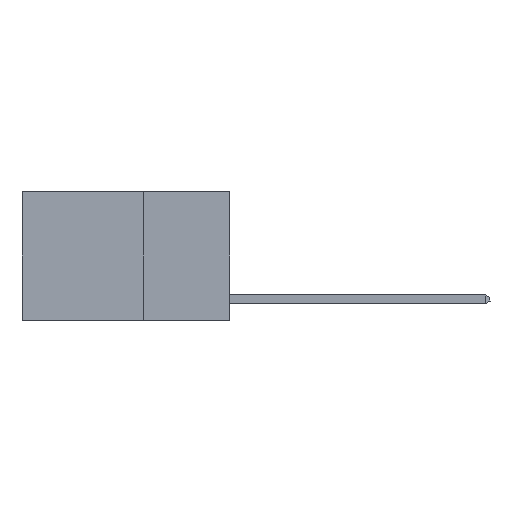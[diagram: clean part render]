
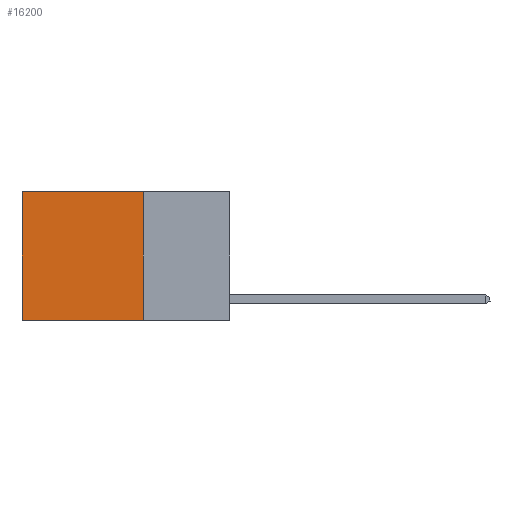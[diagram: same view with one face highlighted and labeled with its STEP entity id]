
A CAD part, left-side view. The second image highlights one B-rep face of the part: STEP entity #16200.
In plain terms, the highlighted planar face has unit normal (-1, 0, 0).
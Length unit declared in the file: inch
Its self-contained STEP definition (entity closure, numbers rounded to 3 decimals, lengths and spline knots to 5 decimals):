
#720 = LINE ( 'NONE', #3498, #6022 ) ;
#1581 = ORIENTED_EDGE ( 'NONE', *, *, #7652, .F. ) ;
#2287 = ORIENTED_EDGE ( 'NONE', *, *, #6703, .T. ) ;
#2832 = DIRECTION ( 'NONE',  ( 0., 0., -1. ) ) ;
#2850 = LINE ( 'NONE', #6928, #14920 ) ;
#2964 = DIRECTION ( 'NONE',  ( 0., 1., 0. ) ) ;
#3498 = CARTESIAN_POINT ( 'NONE',  ( 0.2625, 0.25, -0.37 ) ) ;
#3837 = AXIS2_PLACEMENT_3D ( 'NONE', #6525, #5266, #16897 ) ;
#3869 = CARTESIAN_POINT ( 'NONE',  ( 0.2625, 0.6, 0. ) ) ;
#5266 = DIRECTION ( 'NONE',  ( 1., 0., 0. ) ) ;
#5524 = DIRECTION ( 'NONE',  ( 0., 0., -1. ) ) ;
#5735 = EDGE_CURVE ( 'NONE', #6728, #7796, #10730, .T. ) ;
#5769 = VECTOR ( 'NONE', #2832, 39.37008 ) ;
#6022 = VECTOR ( 'NONE', #8729, 39.37008 ) ;
#6525 = CARTESIAN_POINT ( 'NONE',  ( 0.2625, 0.25, 0. ) ) ;
#6703 = EDGE_CURVE ( 'NONE', #6728, #16732, #8421, .T. ) ;
#6728 = VERTEX_POINT ( 'NONE', #8503 ) ;
#6928 = CARTESIAN_POINT ( 'NONE',  ( 0.2625, 0.6, 0. ) ) ;
#7652 = EDGE_CURVE ( 'NONE', #7796, #8157, #720, .T. ) ;
#7796 = VERTEX_POINT ( 'NONE', #12084 ) ;
#8157 = VERTEX_POINT ( 'NONE', #16683 ) ;
#8421 = LINE ( 'NONE', #14906, #15555 ) ;
#8503 = CARTESIAN_POINT ( 'NONE',  ( 0.2625, 0.25, 0. ) ) ;
#8729 = DIRECTION ( 'NONE',  ( 0., 1., 0. ) ) ;
#9060 = EDGE_CURVE ( 'NONE', #16732, #8157, #2850, .T. ) ;
#10068 = EDGE_LOOP ( 'NONE', ( #13130, #1581, #10437, #2287 ) ) ;
#10246 = FACE_OUTER_BOUND ( 'NONE', #10068, .T. ) ;
#10437 = ORIENTED_EDGE ( 'NONE', *, *, #5735, .F. ) ;
#10730 = LINE ( 'NONE', #13208, #5769 ) ;
#11937 = PLANE ( 'NONE',  #3837 ) ;
#12084 = CARTESIAN_POINT ( 'NONE',  ( 0.2625, 0.25, -0.37 ) ) ;
#13130 = ORIENTED_EDGE ( 'NONE', *, *, #9060, .T. ) ;
#13208 = CARTESIAN_POINT ( 'NONE',  ( 0.2625, 0.25, 0. ) ) ;
#14906 = CARTESIAN_POINT ( 'NONE',  ( 0.2625, 0.25, 0. ) ) ;
#14920 = VECTOR ( 'NONE', #5524, 39.37008 ) ;
#15555 = VECTOR ( 'NONE', #2964, 39.37008 ) ;
#16200 = ADVANCED_FACE ( 'NONE', ( #10246 ), #11937, .F. ) ;
#16683 = CARTESIAN_POINT ( 'NONE',  ( 0.2625, 0.6, -0.37 ) ) ;
#16732 = VERTEX_POINT ( 'NONE', #3869 ) ;
#16897 = DIRECTION ( 'NONE',  ( 0., 0., -1. ) ) ;
